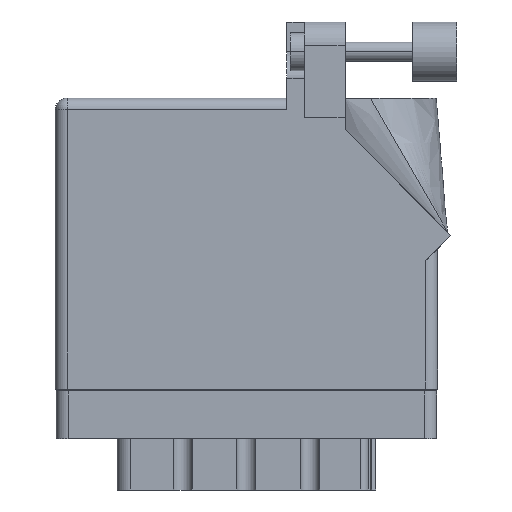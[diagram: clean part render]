
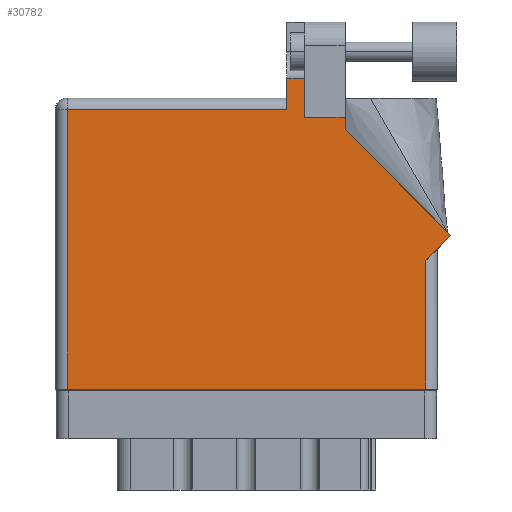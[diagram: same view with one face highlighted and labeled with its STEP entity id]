
A CAD part, front view. The second image highlights one B-rep face of the part: STEP entity #30782.
In plain terms, the highlighted face is planar.
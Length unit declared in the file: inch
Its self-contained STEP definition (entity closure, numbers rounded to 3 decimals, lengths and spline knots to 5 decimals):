
#447 = VECTOR ( 'NONE', #33218, 39.37008 ) ;
#998 = VECTOR ( 'NONE', #11120, 39.37008 ) ;
#1021 = CARTESIAN_POINT ( 'NONE',  ( 1.524, 1.43, 0. ) ) ;
#1469 = PLANE ( 'NONE',  #33051 ) ;
#2699 = EDGE_CURVE ( 'NONE', #22069, #32540, #31089, .T. ) ;
#2847 = LINE ( 'NONE', #31795, #32565 ) ;
#3876 = CARTESIAN_POINT ( 'NONE',  ( 1.948, 0.675, 0. ) ) ;
#4563 = VECTOR ( 'NONE', #40926, 39.37008 ) ;
#4785 = CARTESIAN_POINT ( 'NONE',  ( 1.311, 1.43, 0. ) ) ;
#5826 = LINE ( 'NONE', #27442, #20426 ) ;
#5877 = VECTOR ( 'NONE', #35389, 39.37008 ) ;
#6433 = VECTOR ( 'NONE', #34251, 39.37008 ) ;
#6943 = CARTESIAN_POINT ( 'NONE',  ( 0.062, 0., 0. ) ) ;
#8130 = EDGE_CURVE ( 'NONE', #10011, #33353, #2847, .T. ) ;
#8244 = CARTESIAN_POINT ( 'NONE',  ( 0., 1.468, 0. ) ) ;
#8620 = CARTESIAN_POINT ( 'NONE',  ( 1.524, 1.43, 0. ) ) ;
#8900 = EDGE_LOOP ( 'NONE', ( #16182, #29495, #14614, #21856, #28607, #10680, #31204, #9751, #29608, #34210, #10004 ) ) ;
#9209 = VECTOR ( 'NONE', #37893, 39.37008 ) ;
#9529 = LINE ( 'NONE', #14518, #447 ) ;
#9751 = ORIENTED_EDGE ( 'NONE', *, *, #25996, .T. ) ;
#10004 = ORIENTED_EDGE ( 'NONE', *, *, #39229, .T. ) ;
#10011 = VERTEX_POINT ( 'NONE', #6943 ) ;
#10203 = LINE ( 'NONE', #8620, #9209 ) ;
#10680 = ORIENTED_EDGE ( 'NONE', *, *, #8130, .T. ) ;
#10995 = VECTOR ( 'NONE', #11229, 39.37008 ) ;
#11120 = DIRECTION ( 'NONE',  ( 0., -1., 0. ) ) ;
#11229 = DIRECTION ( 'NONE',  ( 0., 1., 0. ) ) ;
#11813 = VERTEX_POINT ( 'NONE', #12107 ) ;
#12107 = CARTESIAN_POINT ( 'NONE',  ( 1.524, 1.36442, 0. ) ) ;
#14053 = CARTESIAN_POINT ( 'NONE',  ( 1.217, 1.468, 0. ) ) ;
#14518 = CARTESIAN_POINT ( 'NONE',  ( 0.062, 0., 0. ) ) ;
#14614 = ORIENTED_EDGE ( 'NONE', *, *, #33041, .T. ) ;
#14887 = CARTESIAN_POINT ( 'NONE',  ( 1.311, 1.43, 0. ) ) ;
#16182 = ORIENTED_EDGE ( 'NONE', *, *, #33797, .T. ) ;
#17679 = VERTEX_POINT ( 'NONE', #3876 ) ;
#17985 = EDGE_CURVE ( 'NONE', #30563, #29915, #41205, .T. ) ;
#18050 = DIRECTION ( 'NONE',  ( -1., 0., 0. ) ) ;
#20426 = VECTOR ( 'NONE', #31569, 39.37008 ) ;
#20497 = CARTESIAN_POINT ( 'NONE',  ( 1.217, 1.6315, 0. ) ) ;
#20721 = DIRECTION ( 'NONE',  ( 0., 0., -1. ) ) ;
#21393 = DIRECTION ( 'NONE',  ( 0., 1., 0. ) ) ;
#21856 = ORIENTED_EDGE ( 'NONE', *, *, #2699, .T. ) ;
#22069 = VERTEX_POINT ( 'NONE', #14053 ) ;
#22551 = EDGE_CURVE ( 'NONE', #11813, #29309, #25427, .T. ) ;
#22706 = CARTESIAN_POINT ( 'NONE',  ( 1.311, 1.6315, 0. ) ) ;
#24926 = DIRECTION ( 'NONE',  ( -1., 0., 0. ) ) ;
#25427 = LINE ( 'NONE', #32576, #5877 ) ;
#25493 = EDGE_CURVE ( 'NONE', #33353, #17679, #40371, .T. ) ;
#25996 = EDGE_CURVE ( 'NONE', #17679, #36891, #30229, .T. ) ;
#27131 = LINE ( 'NONE', #27252, #998 ) ;
#27192 = EDGE_CURVE ( 'NONE', #32540, #10011, #9529, .T. ) ;
#27252 = CARTESIAN_POINT ( 'NONE',  ( 1.217, 1.53, 0. ) ) ;
#27442 = CARTESIAN_POINT ( 'NONE',  ( 2.08071, 0.80771, 0. ) ) ;
#27825 = FACE_OUTER_BOUND ( 'NONE', #8900, .T. ) ;
#27877 = CARTESIAN_POINT ( 'NONE',  ( 1.64177, 1.6315, 0. ) ) ;
#28118 = CARTESIAN_POINT ( 'NONE',  ( 1.948, 0.737, 0. ) ) ;
#28601 = CARTESIAN_POINT ( 'NONE',  ( 1.948, 0., 0. ) ) ;
#28607 = ORIENTED_EDGE ( 'NONE', *, *, #27192, .T. ) ;
#28932 = EDGE_CURVE ( 'NONE', #36891, #11813, #5826, .T. ) ;
#29108 = LINE ( 'NONE', #4785, #10995 ) ;
#29309 = VERTEX_POINT ( 'NONE', #1021 ) ;
#29495 = ORIENTED_EDGE ( 'NONE', *, *, #17985, .T. ) ;
#29608 = ORIENTED_EDGE ( 'NONE', *, *, #28932, .T. ) ;
#29915 = VERTEX_POINT ( 'NONE', #20497 ) ;
#30229 = LINE ( 'NONE', #34425, #4563 ) ;
#30254 = CARTESIAN_POINT ( 'NONE',  ( 2.08071, 0.80771, 0. ) ) ;
#30563 = VERTEX_POINT ( 'NONE', #22706 ) ;
#30782 = ADVANCED_FACE ( 'NONE', ( #27825 ), #1469, .F. ) ;
#31089 = LINE ( 'NONE', #8244, #6433 ) ;
#31204 = ORIENTED_EDGE ( 'NONE', *, *, #25493, .T. ) ;
#31466 = VERTEX_POINT ( 'NONE', #14887 ) ;
#31569 = DIRECTION ( 'NONE',  ( -0.707, 0.707, 0. ) ) ;
#31795 = CARTESIAN_POINT ( 'NONE',  ( 0., 0., 0. ) ) ;
#31813 = VECTOR ( 'NONE', #21393, 39.37008 ) ;
#32540 = VERTEX_POINT ( 'NONE', #33379 ) ;
#32565 = VECTOR ( 'NONE', #38418, 39.37008 ) ;
#32576 = CARTESIAN_POINT ( 'NONE',  ( 1.524, 1.36442, 0. ) ) ;
#33041 = EDGE_CURVE ( 'NONE', #29915, #22069, #27131, .T. ) ;
#33051 = AXIS2_PLACEMENT_3D ( 'NONE', #33772, #20721, #18050 ) ;
#33218 = DIRECTION ( 'NONE',  ( 0., -1., 0. ) ) ;
#33353 = VERTEX_POINT ( 'NONE', #28601 ) ;
#33379 = CARTESIAN_POINT ( 'NONE',  ( 0.062, 1.468, 0. ) ) ;
#33629 = VECTOR ( 'NONE', #24926, 39.37008 ) ;
#33772 = CARTESIAN_POINT ( 'NONE',  ( 0., 1.53, 0. ) ) ;
#33797 = EDGE_CURVE ( 'NONE', #31466, #30563, #29108, .T. ) ;
#34210 = ORIENTED_EDGE ( 'NONE', *, *, #22551, .T. ) ;
#34251 = DIRECTION ( 'NONE',  ( -1., 0., 0. ) ) ;
#34425 = CARTESIAN_POINT ( 'NONE',  ( 2.01, 0.737, 0. ) ) ;
#35389 = DIRECTION ( 'NONE',  ( 0., 1., 0. ) ) ;
#36891 = VERTEX_POINT ( 'NONE', #30254 ) ;
#37893 = DIRECTION ( 'NONE',  ( -1., 0., 0. ) ) ;
#38418 = DIRECTION ( 'NONE',  ( 1., 0., 0. ) ) ;
#39229 = EDGE_CURVE ( 'NONE', #29309, #31466, #10203, .T. ) ;
#40371 = LINE ( 'NONE', #28118, #31813 ) ;
#40926 = DIRECTION ( 'NONE',  ( 0.707, 0.707, 0. ) ) ;
#41205 = LINE ( 'NONE', #27877, #33629 ) ;
